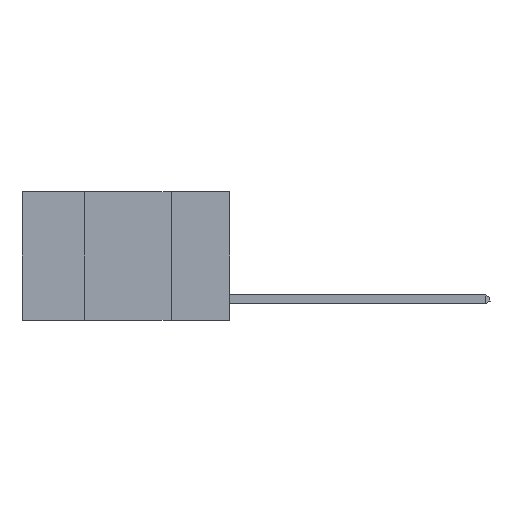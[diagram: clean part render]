
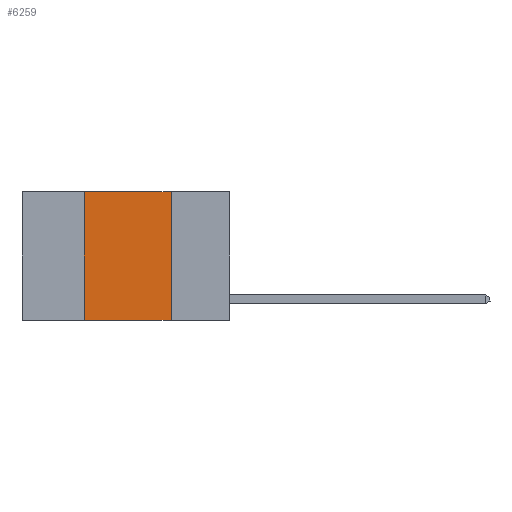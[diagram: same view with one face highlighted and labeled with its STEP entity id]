
A CAD part, left-side view. The second image highlights one B-rep face of the part: STEP entity #6259.
In plain terms, the highlighted planar face has unit normal (-1, 0, 0).
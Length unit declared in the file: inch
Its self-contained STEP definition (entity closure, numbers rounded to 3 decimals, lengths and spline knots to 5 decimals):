
#61 = VERTEX_POINT ( 'NONE', #4823 ) ;
#265 = ORIENTED_EDGE ( 'NONE', *, *, #6326, .F. ) ;
#639 = LINE ( 'NONE', #9002, #10560 ) ;
#735 = EDGE_CURVE ( 'NONE', #5873, #61, #639, .T. ) ;
#834 = VERTEX_POINT ( 'NONE', #9313 ) ;
#990 = VERTEX_POINT ( 'NONE', #14609 ) ;
#1262 = CARTESIAN_POINT ( 'NONE',  ( 0., 0.17, 0. ) ) ;
#2143 = ORIENTED_EDGE ( 'NONE', *, *, #11571, .F. ) ;
#2375 = AXIS2_PLACEMENT_3D ( 'NONE', #3768, #2734, #10807 ) ;
#2734 = DIRECTION ( 'NONE',  ( 1., 0., 0. ) ) ;
#2783 = EDGE_LOOP ( 'NONE', ( #265, #9691, #2143, #8105 ) ) ;
#3496 = CARTESIAN_POINT ( 'NONE',  ( 0., 0.6, -0.37 ) ) ;
#3768 = CARTESIAN_POINT ( 'NONE',  ( 0., 0.6, 0. ) ) ;
#4823 = CARTESIAN_POINT ( 'NONE',  ( 0., 0.17, 0. ) ) ;
#5873 = VERTEX_POINT ( 'NONE', #12220 ) ;
#6259 = ADVANCED_FACE ( 'NONE', ( #9862 ), #10731, .F. ) ;
#6326 = EDGE_CURVE ( 'NONE', #61, #990, #11979, .T. ) ;
#8105 = ORIENTED_EDGE ( 'NONE', *, *, #8321, .T. ) ;
#8321 = EDGE_CURVE ( 'NONE', #834, #990, #9365, .T. ) ;
#9002 = CARTESIAN_POINT ( 'NONE',  ( 0., 0.6, 0. ) ) ;
#9062 = DIRECTION ( 'NONE',  ( 0., 0., -1. ) ) ;
#9313 = CARTESIAN_POINT ( 'NONE',  ( 0., 0.42, -0.37 ) ) ;
#9365 = LINE ( 'NONE', #3496, #12348 ) ;
#9691 = ORIENTED_EDGE ( 'NONE', *, *, #735, .F. ) ;
#9862 = FACE_OUTER_BOUND ( 'NONE', #2783, .T. ) ;
#10292 = LINE ( 'NONE', #15050, #14749 ) ;
#10560 = VECTOR ( 'NONE', #13756, 39.37008 ) ;
#10731 = PLANE ( 'NONE',  #2375 ) ;
#10807 = DIRECTION ( 'NONE',  ( 0., 0., -1. ) ) ;
#11571 = EDGE_CURVE ( 'NONE', #834, #5873, #10292, .T. ) ;
#11629 = DIRECTION ( 'NONE',  ( 0., 0., 1. ) ) ;
#11979 = LINE ( 'NONE', #1262, #12611 ) ;
#12220 = CARTESIAN_POINT ( 'NONE',  ( 0., 0.42, 0. ) ) ;
#12348 = VECTOR ( 'NONE', #15063, 39.37008 ) ;
#12611 = VECTOR ( 'NONE', #9062, 39.37008 ) ;
#13756 = DIRECTION ( 'NONE',  ( 0., -1., 0. ) ) ;
#14609 = CARTESIAN_POINT ( 'NONE',  ( 0., 0.17, -0.37 ) ) ;
#14749 = VECTOR ( 'NONE', #11629, 39.37008 ) ;
#15050 = CARTESIAN_POINT ( 'NONE',  ( 0., 0.42, 0. ) ) ;
#15063 = DIRECTION ( 'NONE',  ( 0., -1., 0. ) ) ;
